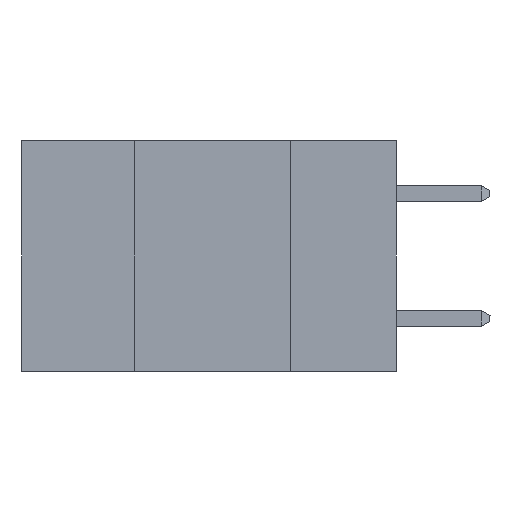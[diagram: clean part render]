
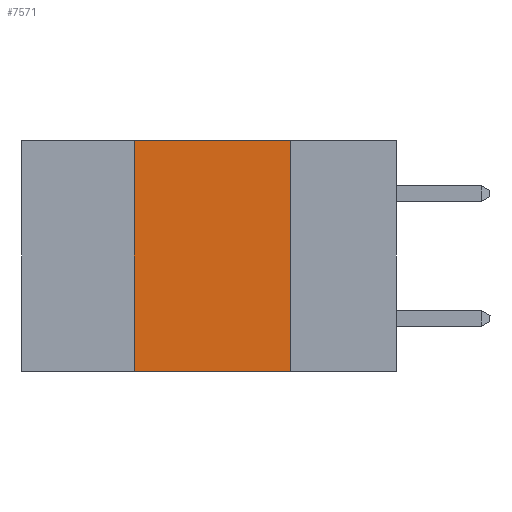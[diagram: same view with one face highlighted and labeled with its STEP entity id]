
A CAD part, left-side view. The second image highlights one B-rep face of the part: STEP entity #7571.
In plain terms, the highlighted planar face has unit normal (-1, 0, 0).
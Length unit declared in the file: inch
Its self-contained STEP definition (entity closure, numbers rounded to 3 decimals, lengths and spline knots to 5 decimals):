
#452 = LINE ( 'NONE', #940, #8266 ) ;
#560 = VECTOR ( 'NONE', #5876, 39.37008 ) ;
#731 = VECTOR ( 'NONE', #3799, 39.37008 ) ;
#940 = CARTESIAN_POINT ( 'NONE',  ( 0., 0.17, -0.37 ) ) ;
#1048 = EDGE_LOOP ( 'NONE', ( #1470, #9639, #1701, #6606 ) ) ;
#1470 = ORIENTED_EDGE ( 'NONE', *, *, #8992, .F. ) ;
#1480 = CARTESIAN_POINT ( 'NONE',  ( 0., 0.42, 0. ) ) ;
#1503 = PLANE ( 'NONE',  #2149 ) ;
#1701 = ORIENTED_EDGE ( 'NONE', *, *, #8727, .F. ) ;
#1985 = EDGE_CURVE ( 'NONE', #8361, #8604, #2962, .T. ) ;
#2149 = AXIS2_PLACEMENT_3D ( 'NONE', #8341, #6796, #2236 ) ;
#2236 = DIRECTION ( 'NONE',  ( 0., 0., -1. ) ) ;
#2274 = DIRECTION ( 'NONE',  ( 0., -1., 0. ) ) ;
#2962 = LINE ( 'NONE', #3880, #731 ) ;
#3454 = CARTESIAN_POINT ( 'NONE',  ( 0., 0.17, 0. ) ) ;
#3583 = CARTESIAN_POINT ( 'NONE',  ( 0., 0.42, -0.37 ) ) ;
#3799 = DIRECTION ( 'NONE',  ( 0., -1., 0. ) ) ;
#3880 = CARTESIAN_POINT ( 'NONE',  ( 0., 0.6, -0.37 ) ) ;
#3928 = VECTOR ( 'NONE', #2274, 39.37008 ) ;
#4415 = VERTEX_POINT ( 'NONE', #1480 ) ;
#4563 = CARTESIAN_POINT ( 'NONE',  ( 0., 0.6, 0. ) ) ;
#4804 = LINE ( 'NONE', #3583, #560 ) ;
#5075 = EDGE_CURVE ( 'NONE', #4415, #9556, #5940, .T. ) ;
#5710 = CARTESIAN_POINT ( 'NONE',  ( 0., 0.17, -0.37 ) ) ;
#5876 = DIRECTION ( 'NONE',  ( 0., 0., 1. ) ) ;
#5940 = LINE ( 'NONE', #4563, #3928 ) ;
#6205 = CARTESIAN_POINT ( 'NONE',  ( 0., 0.42, -0.37 ) ) ;
#6606 = ORIENTED_EDGE ( 'NONE', *, *, #1985, .T. ) ;
#6796 = DIRECTION ( 'NONE',  ( 1., 0., 0. ) ) ;
#7571 = ADVANCED_FACE ( 'NONE', ( #9678 ), #1503, .F. ) ;
#8266 = VECTOR ( 'NONE', #8564, 39.37008 ) ;
#8341 = CARTESIAN_POINT ( 'NONE',  ( 0., 0.6, 0. ) ) ;
#8361 = VERTEX_POINT ( 'NONE', #6205 ) ;
#8564 = DIRECTION ( 'NONE',  ( 0., 0., -1. ) ) ;
#8604 = VERTEX_POINT ( 'NONE', #5710 ) ;
#8727 = EDGE_CURVE ( 'NONE', #8361, #4415, #4804, .T. ) ;
#8992 = EDGE_CURVE ( 'NONE', #9556, #8604, #452, .T. ) ;
#9556 = VERTEX_POINT ( 'NONE', #3454 ) ;
#9639 = ORIENTED_EDGE ( 'NONE', *, *, #5075, .F. ) ;
#9678 = FACE_OUTER_BOUND ( 'NONE', #1048, .T. ) ;
